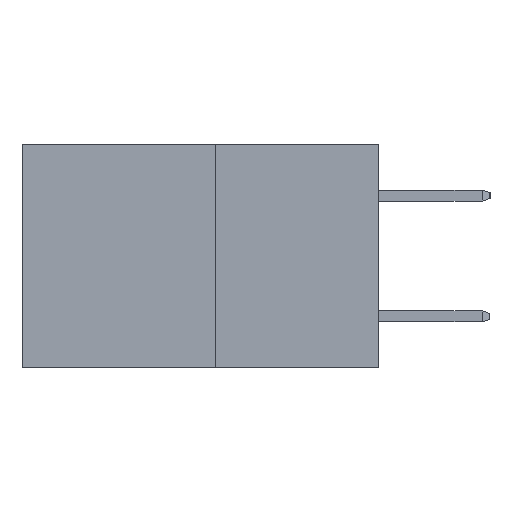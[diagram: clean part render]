
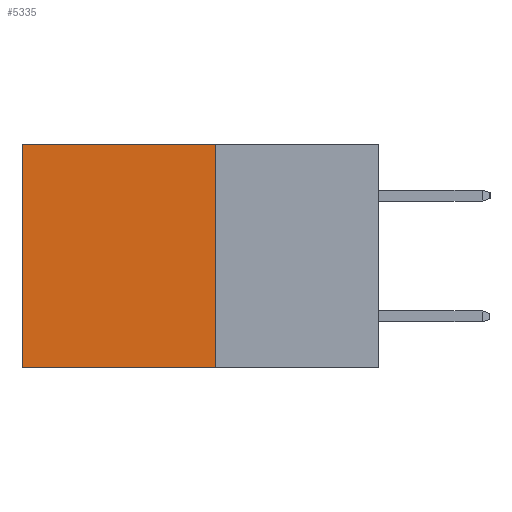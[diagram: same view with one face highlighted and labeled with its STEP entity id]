
A CAD part, left-side view. The second image highlights one B-rep face of the part: STEP entity #5335.
In plain terms, the highlighted planar face has unit normal (-1, 0, 0).
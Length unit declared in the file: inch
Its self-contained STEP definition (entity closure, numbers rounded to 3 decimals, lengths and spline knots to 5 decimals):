
#1 = DIRECTION ( 'NONE',  ( 1., 0., 0. ) ) ;
#255 = VERTEX_POINT ( 'NONE', #2402 ) ;
#700 = CARTESIAN_POINT ( 'NONE',  ( 0.277, 0.27, -0.37 ) ) ;
#2215 = ORIENTED_EDGE ( 'NONE', *, *, #23820, .T. ) ;
#2402 = CARTESIAN_POINT ( 'NONE',  ( 0.277, 0.27, 0. ) ) ;
#3515 = CARTESIAN_POINT ( 'NONE',  ( 0.277, 0.27, 0. ) ) ;
#5043 = VERTEX_POINT ( 'NONE', #13369 ) ;
#5290 = VECTOR ( 'NONE', #12164, 39.37008 ) ;
#5335 = ADVANCED_FACE ( 'NONE', ( #8643 ), #29086, .F. ) ;
#5751 = DIRECTION ( 'NONE',  ( 0., 1., 0. ) ) ;
#6137 = ORIENTED_EDGE ( 'NONE', *, *, #15432, .F. ) ;
#6304 = LINE ( 'NONE', #16831, #17725 ) ;
#7732 = DIRECTION ( 'NONE',  ( 0., 0., -1. ) ) ;
#8643 = FACE_OUTER_BOUND ( 'NONE', #17926, .T. ) ;
#9284 = LINE ( 'NONE', #3515, #26544 ) ;
#9721 = AXIS2_PLACEMENT_3D ( 'NONE', #700, #1, #28907 ) ;
#11217 = LINE ( 'NONE', #14343, #5290 ) ;
#11276 = CARTESIAN_POINT ( 'NONE',  ( 0.277, 0.27, -0.37 ) ) ;
#12164 = DIRECTION ( 'NONE',  ( 0., 0., -1. ) ) ;
#12870 = EDGE_CURVE ( 'NONE', #255, #5043, #9284, .T. ) ;
#13369 = CARTESIAN_POINT ( 'NONE',  ( 0.277, 0.59, 0. ) ) ;
#13393 = VECTOR ( 'NONE', #22601, 39.37008 ) ;
#14343 = CARTESIAN_POINT ( 'NONE',  ( 0.277, 0.59, -0.37 ) ) ;
#14401 = VERTEX_POINT ( 'NONE', #11276 ) ;
#15432 = EDGE_CURVE ( 'NONE', #255, #14401, #6304, .T. ) ;
#16831 = CARTESIAN_POINT ( 'NONE',  ( 0.277, 0.27, -0.37 ) ) ;
#17725 = VECTOR ( 'NONE', #7732, 39.37008 ) ;
#17926 = EDGE_LOOP ( 'NONE', ( #2215, #22592, #6137, #24242 ) ) ;
#19418 = LINE ( 'NONE', #26956, #13393 ) ;
#20267 = CARTESIAN_POINT ( 'NONE',  ( 0.277, 0.59, -0.37 ) ) ;
#21656 = VERTEX_POINT ( 'NONE', #20267 ) ;
#22592 = ORIENTED_EDGE ( 'NONE', *, *, #25677, .F. ) ;
#22601 = DIRECTION ( 'NONE',  ( 0., 1., 0. ) ) ;
#23820 = EDGE_CURVE ( 'NONE', #5043, #21656, #11217, .T. ) ;
#24242 = ORIENTED_EDGE ( 'NONE', *, *, #12870, .T. ) ;
#25677 = EDGE_CURVE ( 'NONE', #14401, #21656, #19418, .T. ) ;
#26544 = VECTOR ( 'NONE', #5751, 39.37008 ) ;
#26956 = CARTESIAN_POINT ( 'NONE',  ( 0.277, 0.27, -0.37 ) ) ;
#28907 = DIRECTION ( 'NONE',  ( 0., 0., -1. ) ) ;
#29086 = PLANE ( 'NONE',  #9721 ) ;
